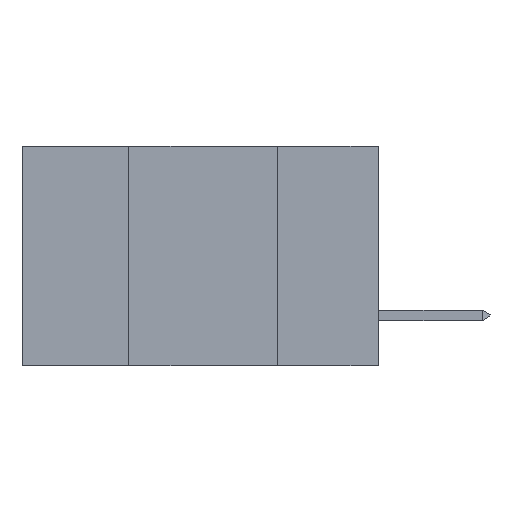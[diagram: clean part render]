
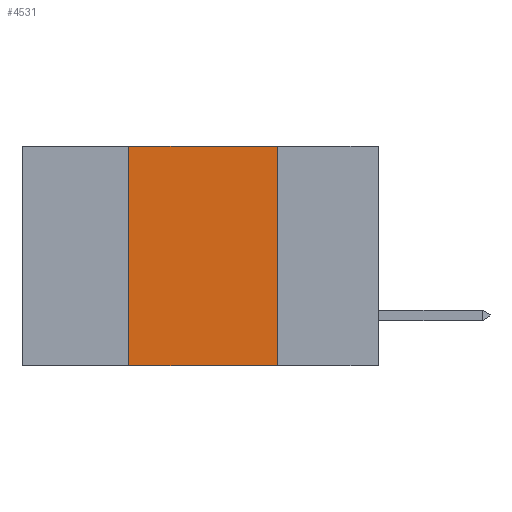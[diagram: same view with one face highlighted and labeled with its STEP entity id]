
A CAD part, left-side view. The second image highlights one B-rep face of the part: STEP entity #4531.
In plain terms, the highlighted planar face has unit normal (-1, 0, 0).
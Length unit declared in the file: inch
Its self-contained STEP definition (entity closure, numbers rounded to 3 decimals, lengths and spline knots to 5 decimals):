
#1429 = CARTESIAN_POINT ( 'NONE',  ( 0., 0.17, 0. ) ) ;
#1801 = CARTESIAN_POINT ( 'NONE',  ( 0., 0.42, 0. ) ) ;
#3915 = ORIENTED_EDGE ( 'NONE', *, *, #16078, .F. ) ;
#4059 = LINE ( 'NONE', #16678, #5809 ) ;
#4261 = EDGE_CURVE ( 'NONE', #6959, #15478, #17176, .T. ) ;
#4324 = DIRECTION ( 'NONE',  ( 0., 0., -1. ) ) ;
#4531 = ADVANCED_FACE ( 'NONE', ( #7196 ), #12450, .F. ) ;
#4673 = CARTESIAN_POINT ( 'NONE',  ( 0., 0.42, 0. ) ) ;
#4847 = DIRECTION ( 'NONE',  ( 0., 0., 1. ) ) ;
#5466 = CARTESIAN_POINT ( 'NONE',  ( 0., 0.17, -0.37 ) ) ;
#5809 = VECTOR ( 'NONE', #5866, 39.37008 ) ;
#5866 = DIRECTION ( 'NONE',  ( 0., -1., 0. ) ) ;
#5920 = VECTOR ( 'NONE', #4324, 39.37008 ) ;
#6139 = EDGE_CURVE ( 'NONE', #6959, #11084, #8736, .T. ) ;
#6959 = VERTEX_POINT ( 'NONE', #14933 ) ;
#7196 = FACE_OUTER_BOUND ( 'NONE', #15675, .T. ) ;
#7850 = VECTOR ( 'NONE', #16426, 39.37008 ) ;
#8561 = ORIENTED_EDGE ( 'NONE', *, *, #6139, .T. ) ;
#8596 = AXIS2_PLACEMENT_3D ( 'NONE', #15369, #16786, #12569 ) ;
#8733 = VECTOR ( 'NONE', #4847, 39.37008 ) ;
#8736 = LINE ( 'NONE', #13702, #7850 ) ;
#9582 = EDGE_CURVE ( 'NONE', #15478, #17370, #4059, .T. ) ;
#11084 = VERTEX_POINT ( 'NONE', #5466 ) ;
#12450 = PLANE ( 'NONE',  #8596 ) ;
#12558 = CARTESIAN_POINT ( 'NONE',  ( 0., 0.17, 0. ) ) ;
#12569 = DIRECTION ( 'NONE',  ( 0., 0., -1. ) ) ;
#13641 = ORIENTED_EDGE ( 'NONE', *, *, #9582, .F. ) ;
#13702 = CARTESIAN_POINT ( 'NONE',  ( 0., 0.6, -0.37 ) ) ;
#14933 = CARTESIAN_POINT ( 'NONE',  ( 0., 0.42, -0.37 ) ) ;
#15369 = CARTESIAN_POINT ( 'NONE',  ( 0., 0.6, 0. ) ) ;
#15478 = VERTEX_POINT ( 'NONE', #1801 ) ;
#15675 = EDGE_LOOP ( 'NONE', ( #3915, #13641, #17652, #8561 ) ) ;
#16078 = EDGE_CURVE ( 'NONE', #17370, #11084, #16984, .T. ) ;
#16426 = DIRECTION ( 'NONE',  ( 0., -1., 0. ) ) ;
#16678 = CARTESIAN_POINT ( 'NONE',  ( 0., 0.6, 0. ) ) ;
#16786 = DIRECTION ( 'NONE',  ( 1., 0., 0. ) ) ;
#16984 = LINE ( 'NONE', #1429, #5920 ) ;
#17176 = LINE ( 'NONE', #4673, #8733 ) ;
#17370 = VERTEX_POINT ( 'NONE', #12558 ) ;
#17652 = ORIENTED_EDGE ( 'NONE', *, *, #4261, .F. ) ;
